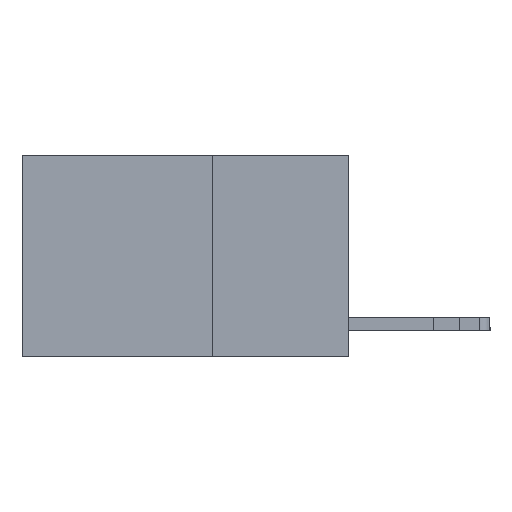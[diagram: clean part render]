
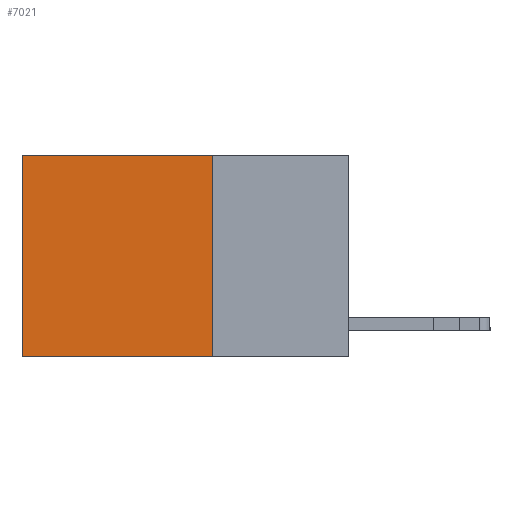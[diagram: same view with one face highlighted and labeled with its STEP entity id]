
A CAD part, left-side view. The second image highlights one B-rep face of the part: STEP entity #7021.
In plain terms, the highlighted planar face has unit normal (-1, 0, 0).
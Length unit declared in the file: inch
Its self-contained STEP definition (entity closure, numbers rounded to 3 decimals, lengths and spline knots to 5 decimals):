
#115 = VECTOR ( 'NONE', #3433, 39.37008 ) ;
#262 = CARTESIAN_POINT ( 'NONE',  ( 0.2625, 0.25, 0. ) ) ;
#497 = DIRECTION ( 'NONE',  ( 0., 1., 0. ) ) ;
#643 = CARTESIAN_POINT ( 'NONE',  ( 0.2625, 0.6, 0. ) ) ;
#752 = DIRECTION ( 'NONE',  ( 0., 0., -1. ) ) ;
#1268 = EDGE_LOOP ( 'NONE', ( #4941, #3314, #12959, #9695 ) ) ;
#1830 = DIRECTION ( 'NONE',  ( 1., 0., 0. ) ) ;
#1898 = CARTESIAN_POINT ( 'NONE',  ( 0.2625, 0.25, 0. ) ) ;
#3304 = AXIS2_PLACEMENT_3D ( 'NONE', #1898, #1830, #752 ) ;
#3314 = ORIENTED_EDGE ( 'NONE', *, *, #12994, .F. ) ;
#3433 = DIRECTION ( 'NONE',  ( 0., 1., 0. ) ) ;
#4941 = ORIENTED_EDGE ( 'NONE', *, *, #7824, .T. ) ;
#5007 = DIRECTION ( 'NONE',  ( 0., 0., -1. ) ) ;
#5348 = VECTOR ( 'NONE', #5007, 39.37008 ) ;
#5732 = VERTEX_POINT ( 'NONE', #262 ) ;
#6401 = FACE_OUTER_BOUND ( 'NONE', #1268, .T. ) ;
#6481 = EDGE_CURVE ( 'NONE', #5732, #13925, #10478, .T. ) ;
#6614 = CARTESIAN_POINT ( 'NONE',  ( 0.2625, 0.25, 0. ) ) ;
#6778 = LINE ( 'NONE', #7912, #12186 ) ;
#6953 = CARTESIAN_POINT ( 'NONE',  ( 0.2625, 0.6, -0.37 ) ) ;
#7021 = ADVANCED_FACE ( 'NONE', ( #6401 ), #12799, .F. ) ;
#7824 = EDGE_CURVE ( 'NONE', #13925, #8610, #8352, .T. ) ;
#7912 = CARTESIAN_POINT ( 'NONE',  ( 0.2625, 0.25, -0.37 ) ) ;
#8352 = LINE ( 'NONE', #643, #5348 ) ;
#8610 = VERTEX_POINT ( 'NONE', #6953 ) ;
#9695 = ORIENTED_EDGE ( 'NONE', *, *, #6481, .T. ) ;
#9761 = EDGE_CURVE ( 'NONE', #5732, #11810, #12040, .T. ) ;
#9890 = DIRECTION ( 'NONE',  ( 0., 0., -1. ) ) ;
#10133 = CARTESIAN_POINT ( 'NONE',  ( 0.2625, 0.25, 0. ) ) ;
#10478 = LINE ( 'NONE', #10133, #115 ) ;
#11282 = VECTOR ( 'NONE', #9890, 39.37008 ) ;
#11810 = VERTEX_POINT ( 'NONE', #12785 ) ;
#12040 = LINE ( 'NONE', #6614, #11282 ) ;
#12186 = VECTOR ( 'NONE', #497, 39.37008 ) ;
#12785 = CARTESIAN_POINT ( 'NONE',  ( 0.2625, 0.25, -0.37 ) ) ;
#12799 = PLANE ( 'NONE',  #3304 ) ;
#12959 = ORIENTED_EDGE ( 'NONE', *, *, #9761, .F. ) ;
#12994 = EDGE_CURVE ( 'NONE', #11810, #8610, #6778, .T. ) ;
#13631 = CARTESIAN_POINT ( 'NONE',  ( 0.2625, 0.6, 0. ) ) ;
#13925 = VERTEX_POINT ( 'NONE', #13631 ) ;
